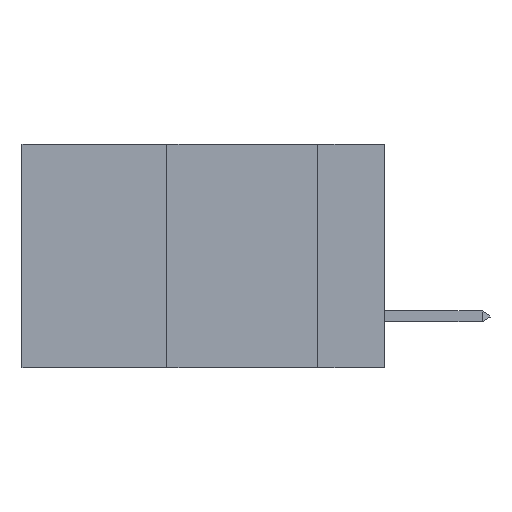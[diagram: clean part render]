
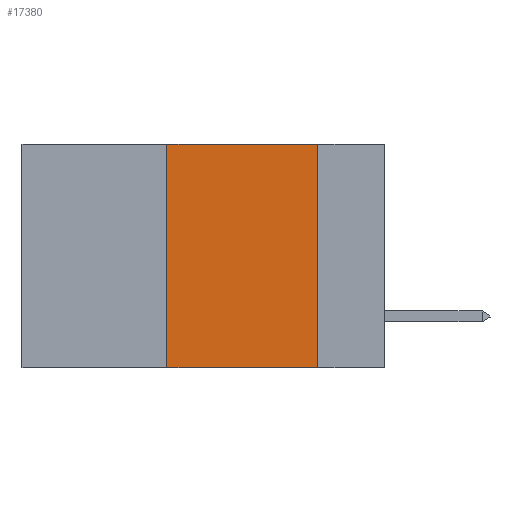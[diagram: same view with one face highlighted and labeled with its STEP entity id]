
A CAD part, left-side view. The second image highlights one B-rep face of the part: STEP entity #17380.
In plain terms, the highlighted planar face has unit normal (-1, 0, 0).
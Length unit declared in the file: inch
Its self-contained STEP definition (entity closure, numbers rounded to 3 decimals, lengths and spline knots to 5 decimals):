
#638 = LINE ( 'NONE', #16177, #1589 ) ;
#1095 = CARTESIAN_POINT ( 'NONE',  ( 0., 0.36, -0.37 ) ) ;
#1589 = VECTOR ( 'NONE', #6655, 39.37008 ) ;
#2690 = VERTEX_POINT ( 'NONE', #17251 ) ;
#2693 = VERTEX_POINT ( 'NONE', #24942 ) ;
#3633 = EDGE_CURVE ( 'NONE', #17150, #2693, #19031, .T. ) ;
#5341 = EDGE_CURVE ( 'NONE', #13337, #2690, #19789, .T. ) ;
#5939 = CARTESIAN_POINT ( 'NONE',  ( 0., 0.36, 0. ) ) ;
#6103 = FACE_OUTER_BOUND ( 'NONE', #20747, .T. ) ;
#6655 = DIRECTION ( 'NONE',  ( 0., 0., -1. ) ) ;
#7270 = VECTOR ( 'NONE', #23291, 39.37008 ) ;
#7448 = CARTESIAN_POINT ( 'NONE',  ( 0., 0.6, 0. ) ) ;
#7480 = VECTOR ( 'NONE', #9307, 39.37008 ) ;
#9307 = DIRECTION ( 'NONE',  ( 0., -1., 0. ) ) ;
#11302 = DIRECTION ( 'NONE',  ( 1., 0., 0. ) ) ;
#12075 = ORIENTED_EDGE ( 'NONE', *, *, #24722, .F. ) ;
#13337 = VERTEX_POINT ( 'NONE', #1095 ) ;
#13342 = CARTESIAN_POINT ( 'NONE',  ( 0., 0.6, 0. ) ) ;
#14733 = CARTESIAN_POINT ( 'NONE',  ( 0., 0.36, 0. ) ) ;
#14825 = DIRECTION ( 'NONE',  ( 0., 0., -1. ) ) ;
#15097 = PLANE ( 'NONE',  #15925 ) ;
#15100 = ORIENTED_EDGE ( 'NONE', *, *, #17097, .F. ) ;
#15220 = CARTESIAN_POINT ( 'NONE',  ( 0., 0.6, -0.37 ) ) ;
#15925 = AXIS2_PLACEMENT_3D ( 'NONE', #7448, #11302, #14825 ) ;
#16177 = CARTESIAN_POINT ( 'NONE',  ( 0., 0.11, 0. ) ) ;
#17097 = EDGE_CURVE ( 'NONE', #2693, #2690, #638, .T. ) ;
#17150 = VERTEX_POINT ( 'NONE', #14733 ) ;
#17251 = CARTESIAN_POINT ( 'NONE',  ( 0., 0.11, -0.37 ) ) ;
#17380 = ADVANCED_FACE ( 'NONE', ( #6103 ), #15097, .F. ) ;
#17723 = DIRECTION ( 'NONE',  ( 0., 0., 1. ) ) ;
#19031 = LINE ( 'NONE', #13342, #7270 ) ;
#19340 = LINE ( 'NONE', #5939, #22964 ) ;
#19789 = LINE ( 'NONE', #15220, #7480 ) ;
#20154 = ORIENTED_EDGE ( 'NONE', *, *, #5341, .T. ) ;
#20747 = EDGE_LOOP ( 'NONE', ( #15100, #24128, #12075, #20154 ) ) ;
#22964 = VECTOR ( 'NONE', #17723, 39.37008 ) ;
#23291 = DIRECTION ( 'NONE',  ( 0., -1., 0. ) ) ;
#24128 = ORIENTED_EDGE ( 'NONE', *, *, #3633, .F. ) ;
#24722 = EDGE_CURVE ( 'NONE', #13337, #17150, #19340, .T. ) ;
#24942 = CARTESIAN_POINT ( 'NONE',  ( 0., 0.11, 0. ) ) ;
